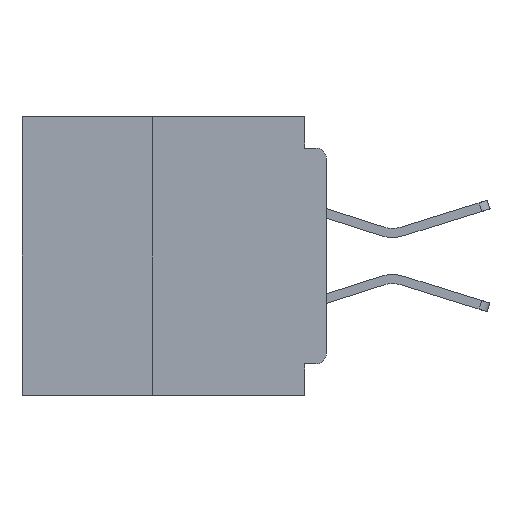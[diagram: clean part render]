
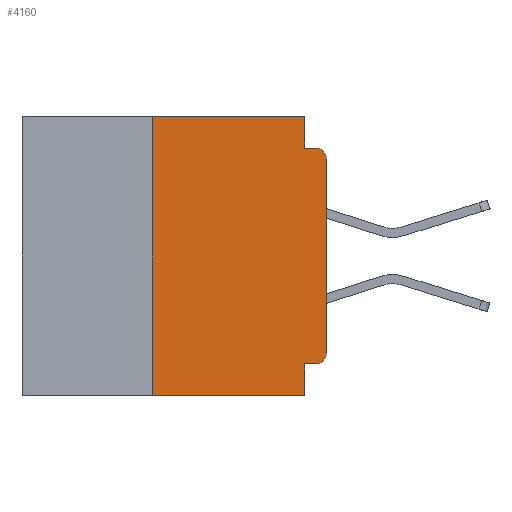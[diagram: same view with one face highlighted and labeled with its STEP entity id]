
A CAD part, left-side view. The second image highlights one B-rep face of the part: STEP entity #4160.
In plain terms, the highlighted planar face has unit normal (-1, 0, 0).
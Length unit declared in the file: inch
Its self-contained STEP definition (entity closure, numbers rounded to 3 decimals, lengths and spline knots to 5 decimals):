
#697 = CARTESIAN_POINT ( 'NONE',  ( 0., 0., -0.06 ) ) ;
#1924 = ORIENTED_EDGE ( 'NONE', *, *, #20646, .T. ) ;
#2885 = EDGE_CURVE ( 'NONE', #28756, #55415, #19689, .T. ) ;
#3386 = VECTOR ( 'NONE', #24590, 39.37008 ) ;
#3493 = EDGE_CURVE ( 'NONE', #56082, #12700, #12686, .T. ) ;
#3691 = DIRECTION ( 'NONE',  ( 0., -1., 0. ) ) ;
#3699 = VERTEX_POINT ( 'NONE', #50168 ) ;
#4138 = ORIENTED_EDGE ( 'NONE', *, *, #47504, .F. ) ;
#4160 = ADVANCED_FACE ( 'NONE', ( #14697 ), #36219, .F. ) ;
#4456 = CARTESIAN_POINT ( 'NONE',  ( 0., 0.437, 0. ) ) ;
#5046 = CARTESIAN_POINT ( 'NONE',  ( 0., 0.031, 0. ) ) ;
#7053 = VERTEX_POINT ( 'NONE', #7782 ) ;
#7118 = CARTESIAN_POINT ( 'NONE',  ( 0., 0.015, -0.06 ) ) ;
#7653 = DIRECTION ( 'NONE',  ( 0., 0., -1. ) ) ;
#7782 = CARTESIAN_POINT ( 'NONE',  ( 0., 0.25, -0.4 ) ) ;
#8464 = VERTEX_POINT ( 'NONE', #47228 ) ;
#9709 = VECTOR ( 'NONE', #16804, 39.37008 ) ;
#9953 = CARTESIAN_POINT ( 'NONE',  ( 0., 0.437, -0.4 ) ) ;
#11513 = DIRECTION ( 'NONE',  ( 0., 0., -1. ) ) ;
#11767 = EDGE_CURVE ( 'NONE', #50463, #33622, #41820, .T. ) ;
#11907 = DIRECTION ( 'NONE',  ( 0., 0., 1. ) ) ;
#12415 = ORIENTED_EDGE ( 'NONE', *, *, #3493, .F. ) ;
#12686 = LINE ( 'NONE', #4456, #34596 ) ;
#12700 = VERTEX_POINT ( 'NONE', #5046 ) ;
#12728 = LINE ( 'NONE', #36404, #46078 ) ;
#14398 = DIRECTION ( 'NONE',  ( 0., -1., 0. ) ) ;
#14697 = FACE_OUTER_BOUND ( 'NONE', #45277, .T. ) ;
#16021 = CARTESIAN_POINT ( 'NONE',  ( 0., 0.015, -0.34 ) ) ;
#16804 = DIRECTION ( 'NONE',  ( 0., 1., 0. ) ) ;
#16817 = CARTESIAN_POINT ( 'NONE',  ( 0., 0., -0.045 ) ) ;
#18044 = ORIENTED_EDGE ( 'NONE', *, *, #11767, .F. ) ;
#18045 = EDGE_CURVE ( 'NONE', #8464, #28756, #30596, .T. ) ;
#19689 = LINE ( 'NONE', #56312, #21048 ) ;
#20429 = DIRECTION ( 'NONE',  ( 0., 0., -1. ) ) ;
#20646 = EDGE_CURVE ( 'NONE', #7053, #33622, #37518, .T. ) ;
#21048 = VECTOR ( 'NONE', #11907, 39.37008 ) ;
#22656 = ORIENTED_EDGE ( 'NONE', *, *, #52843, .F. ) ;
#23909 = EDGE_CURVE ( 'NONE', #55415, #52728, #26255, .T. ) ;
#24590 = DIRECTION ( 'NONE',  ( 0., 0., 1. ) ) ;
#26255 = CIRCLE ( 'NONE', #54193, 0.015 ) ;
#26257 = CARTESIAN_POINT ( 'NONE',  ( 0., 0.031, -0.4 ) ) ;
#26780 = LINE ( 'NONE', #41645, #3386 ) ;
#27380 = ORIENTED_EDGE ( 'NONE', *, *, #2885, .T. ) ;
#28350 = AXIS2_PLACEMENT_3D ( 'NONE', #16021, #46358, #20429 ) ;
#28756 = VERTEX_POINT ( 'NONE', #45747 ) ;
#30596 = CIRCLE ( 'NONE', #28350, 0.015 ) ;
#33622 = VERTEX_POINT ( 'NONE', #26257 ) ;
#33880 = CARTESIAN_POINT ( 'NONE',  ( 0., 0.031, -0.4 ) ) ;
#34341 = CARTESIAN_POINT ( 'NONE',  ( 0., 0., -0.355 ) ) ;
#34373 = LINE ( 'NONE', #34341, #9709 ) ;
#34596 = VECTOR ( 'NONE', #44296, 39.37008 ) ;
#36024 = DIRECTION ( 'NONE',  ( 0., 0., -1. ) ) ;
#36032 = DIRECTION ( 'NONE',  ( 1., 0., 0. ) ) ;
#36101 = CARTESIAN_POINT ( 'NONE',  ( 0., 0.437, 0. ) ) ;
#36164 = VECTOR ( 'NONE', #14398, 39.37008 ) ;
#36219 = PLANE ( 'NONE',  #39388 ) ;
#36404 = CARTESIAN_POINT ( 'NONE',  ( 0., 0.031, 0. ) ) ;
#37518 = LINE ( 'NONE', #9953, #36164 ) ;
#37690 = DIRECTION ( 'NONE',  ( -1., 0., 0. ) ) ;
#38108 = EDGE_CURVE ( 'NONE', #7053, #56082, #26780, .T. ) ;
#38565 = ORIENTED_EDGE ( 'NONE', *, *, #18045, .T. ) ;
#39388 = AXIS2_PLACEMENT_3D ( 'NONE', #36101, #36032, #36024 ) ;
#40796 = CARTESIAN_POINT ( 'NONE',  ( 0., 0.25, 0. ) ) ;
#40903 = DIRECTION ( 'NONE',  ( 0., 0., -1. ) ) ;
#41645 = CARTESIAN_POINT ( 'NONE',  ( 0., 0.25, -0.4 ) ) ;
#41820 = LINE ( 'NONE', #33880, #53227 ) ;
#44296 = DIRECTION ( 'NONE',  ( 0., -1., 0. ) ) ;
#45277 = EDGE_LOOP ( 'NONE', ( #27380, #54645, #55351, #4138, #12415, #48518, #1924, #18044, #22656, #38565 ) ) ;
#45747 = CARTESIAN_POINT ( 'NONE',  ( 0., 0., -0.34 ) ) ;
#46078 = VECTOR ( 'NONE', #40903, 39.37008 ) ;
#46337 = CARTESIAN_POINT ( 'NONE',  ( 0., 0.031, -0.355 ) ) ;
#46358 = DIRECTION ( 'NONE',  ( -1., 0., 0. ) ) ;
#47228 = CARTESIAN_POINT ( 'NONE',  ( 0., 0.015, -0.355 ) ) ;
#47504 = EDGE_CURVE ( 'NONE', #12700, #3699, #12728, .T. ) ;
#48518 = ORIENTED_EDGE ( 'NONE', *, *, #38108, .F. ) ;
#50168 = CARTESIAN_POINT ( 'NONE',  ( 0., 0.031, -0.045 ) ) ;
#50290 = VECTOR ( 'NONE', #3691, 39.37008 ) ;
#50463 = VERTEX_POINT ( 'NONE', #46337 ) ;
#50711 = CARTESIAN_POINT ( 'NONE',  ( 0., 0.015, -0.045 ) ) ;
#51636 = LINE ( 'NONE', #16817, #50290 ) ;
#52728 = VERTEX_POINT ( 'NONE', #50711 ) ;
#52843 = EDGE_CURVE ( 'NONE', #8464, #50463, #34373, .T. ) ;
#53227 = VECTOR ( 'NONE', #7653, 39.37008 ) ;
#54193 = AXIS2_PLACEMENT_3D ( 'NONE', #7118, #37690, #11513 ) ;
#54627 = EDGE_CURVE ( 'NONE', #3699, #52728, #51636, .T. ) ;
#54645 = ORIENTED_EDGE ( 'NONE', *, *, #23909, .T. ) ;
#55351 = ORIENTED_EDGE ( 'NONE', *, *, #54627, .F. ) ;
#55415 = VERTEX_POINT ( 'NONE', #697 ) ;
#56082 = VERTEX_POINT ( 'NONE', #40796 ) ;
#56312 = CARTESIAN_POINT ( 'NONE',  ( 0., 0., 0. ) ) ;
